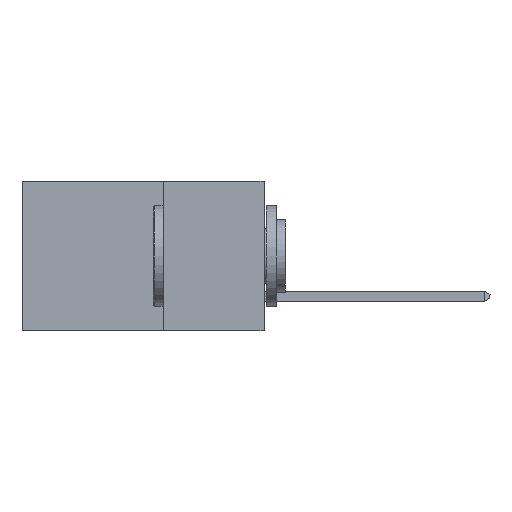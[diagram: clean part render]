
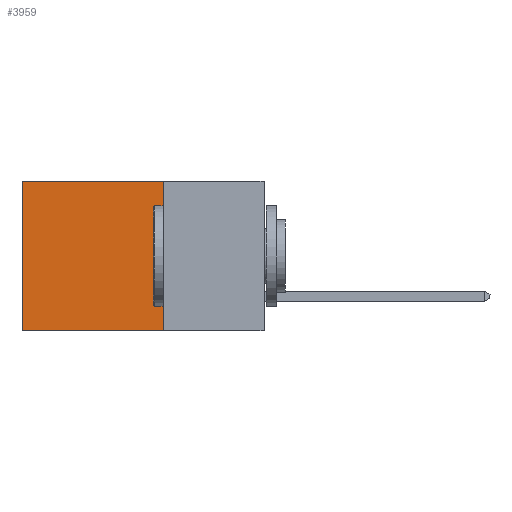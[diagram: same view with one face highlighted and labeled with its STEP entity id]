
A CAD part, left-side view. The second image highlights one B-rep face of the part: STEP entity #3959.
In plain terms, the highlighted planar face has unit normal (-1, 0, 0).
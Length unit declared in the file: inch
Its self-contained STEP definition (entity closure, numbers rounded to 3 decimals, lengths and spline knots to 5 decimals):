
#372 = AXIS2_PLACEMENT_3D ( 'NONE', #8687, #611, #1517 ) ;
#611 = DIRECTION ( 'NONE',  ( 1., 0., 0. ) ) ;
#702 = VERTEX_POINT ( 'NONE', #5484 ) ;
#1084 = EDGE_CURVE ( 'NONE', #702, #4792, #6137, .T. ) ;
#1141 = LINE ( 'NONE', #5566, #5432 ) ;
#1310 = EDGE_CURVE ( 'NONE', #7661, #702, #6645, .T. ) ;
#1453 = CARTESIAN_POINT ( 'NONE',  ( 0.2615, 0.25, 0. ) ) ;
#1465 = DIRECTION ( 'NONE',  ( 0., 0., -1. ) ) ;
#1517 = DIRECTION ( 'NONE',  ( 0., 0., -1. ) ) ;
#2521 = EDGE_CURVE ( 'NONE', #3088, #4792, #1141, .T. ) ;
#2778 = FACE_OUTER_BOUND ( 'NONE', #4684, .T. ) ;
#2818 = CARTESIAN_POINT ( 'NONE',  ( 0.2615, 0.6, -0.37 ) ) ;
#2951 = VECTOR ( 'NONE', #9064, 39.37008 ) ;
#3088 = VERTEX_POINT ( 'NONE', #3498 ) ;
#3498 = CARTESIAN_POINT ( 'NONE',  ( 0.2615, 0.25, -0.37 ) ) ;
#3744 = LINE ( 'NONE', #8906, #4559 ) ;
#3959 = ADVANCED_FACE ( 'NONE', ( #2778 ), #8013, .F. ) ;
#4157 = ORIENTED_EDGE ( 'NONE', *, *, #1310, .T. ) ;
#4559 = VECTOR ( 'NONE', #1465, 39.37008 ) ;
#4684 = EDGE_LOOP ( 'NONE', ( #5691, #9369, #8027, #4157 ) ) ;
#4792 = VERTEX_POINT ( 'NONE', #2818 ) ;
#5117 = CARTESIAN_POINT ( 'NONE',  ( 0.2615, 0.25, 0. ) ) ;
#5432 = VECTOR ( 'NONE', #8497, 39.37008 ) ;
#5484 = CARTESIAN_POINT ( 'NONE',  ( 0.2615, 0.6, 0. ) ) ;
#5566 = CARTESIAN_POINT ( 'NONE',  ( 0.2615, 0.25, -0.37 ) ) ;
#5691 = ORIENTED_EDGE ( 'NONE', *, *, #1084, .T. ) ;
#5949 = CARTESIAN_POINT ( 'NONE',  ( 0.2615, 0.6, -0.37 ) ) ;
#6137 = LINE ( 'NONE', #5949, #2951 ) ;
#6645 = LINE ( 'NONE', #5117, #9080 ) ;
#7276 = EDGE_CURVE ( 'NONE', #7661, #3088, #3744, .T. ) ;
#7661 = VERTEX_POINT ( 'NONE', #1453 ) ;
#8013 = PLANE ( 'NONE',  #372 ) ;
#8027 = ORIENTED_EDGE ( 'NONE', *, *, #7276, .F. ) ;
#8042 = DIRECTION ( 'NONE',  ( 0., 1., 0. ) ) ;
#8497 = DIRECTION ( 'NONE',  ( 0., 1., 0. ) ) ;
#8687 = CARTESIAN_POINT ( 'NONE',  ( 0.2615, 0.25, -0.37 ) ) ;
#8906 = CARTESIAN_POINT ( 'NONE',  ( 0.2615, 0.25, -0.37 ) ) ;
#9064 = DIRECTION ( 'NONE',  ( 0., 0., -1. ) ) ;
#9080 = VECTOR ( 'NONE', #8042, 39.37008 ) ;
#9369 = ORIENTED_EDGE ( 'NONE', *, *, #2521, .F. ) ;
